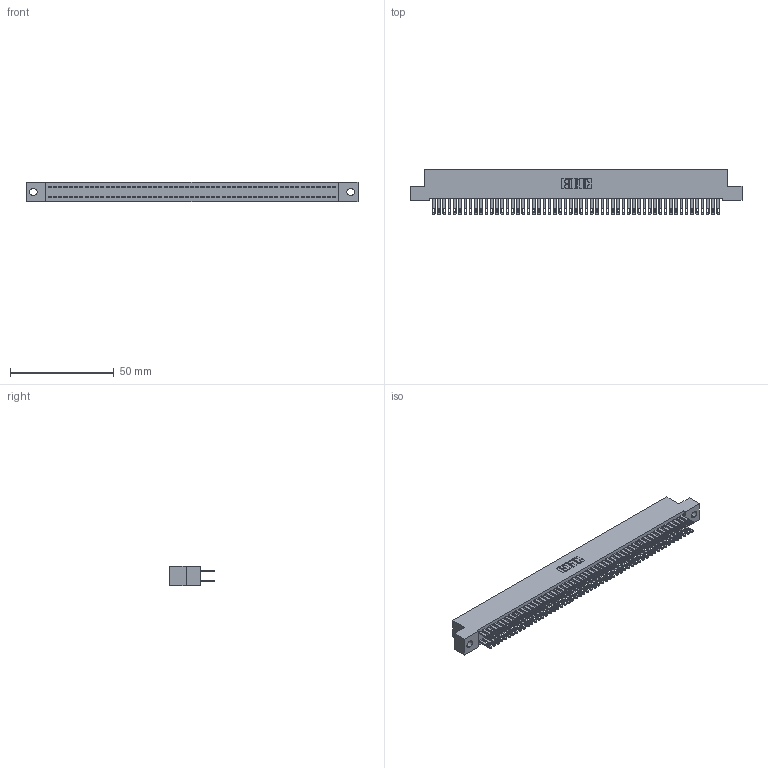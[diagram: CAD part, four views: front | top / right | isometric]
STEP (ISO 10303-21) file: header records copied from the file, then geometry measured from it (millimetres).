
FILE_DESCRIPTION (( 'STEP AP203' ), '1' );
FILE_NAME ('342-110-500-202.STEP', '2019-10-04T20:06:45', ( '' ), ( '' ), 'SwSTEP 2.0', 'SolidWorks 2016', '' );
FILE_SCHEMA (( 'CONFIG_CONTROL_DESIGN' ));
Length unit declared in the file: inch
Products named in the file (3): 345-292-001_345-293-100; 342-110-500-202; 342 Part_.128 Slot
Assembly tree (111 placements, depth 2):
  342-110-500-202
    342 Part_.128 Slot
    345-292-001_345-293-100  x110
Bounding box: 160.02 x 21.85 x 9.4 mm (x, y, z)
Volume: 14723.3 mm3; surface area: 25098.9 mm2
Topology: 111 solids, 111 shells, 5394 faces, 16481 edges, 10986 vertices
Faces by surface type: plane 3370, cylinder 2024
Entity records: 33635 total; most frequent: CARTESIAN_POINT 5558, ORIENTED_EDGE 5494, DIRECTION 4727, EDGE_CURVE 2747, LINE 2615, VECTOR 2615, VERTEX_POINT 1830, AXIS2_PLACEMENT_3D 1056
